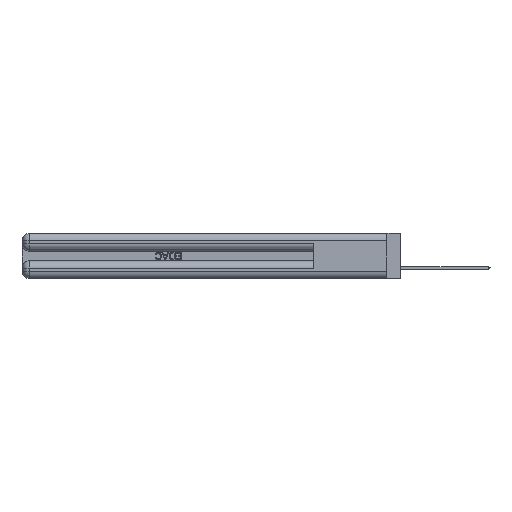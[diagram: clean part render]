
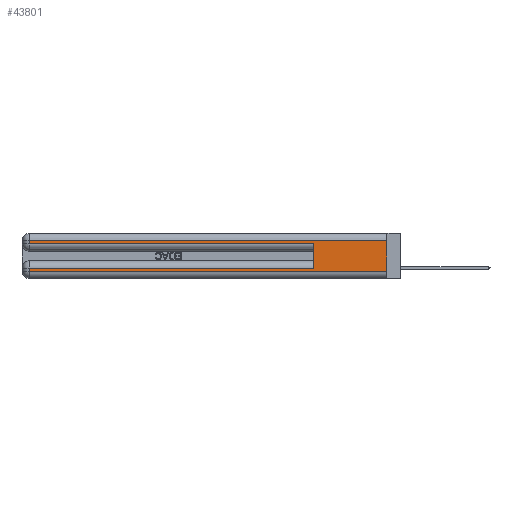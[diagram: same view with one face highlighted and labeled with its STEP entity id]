
A CAD part, left-side view. The second image highlights one B-rep face of the part: STEP entity #43801.
In plain terms, the highlighted planar face has unit normal (-1, 0, 0).
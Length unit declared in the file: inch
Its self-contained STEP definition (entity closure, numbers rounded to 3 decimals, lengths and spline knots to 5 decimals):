
#1832 = DIRECTION ( 'NONE',  ( 0., -1., 0. ) ) ;
#1915 = DIRECTION ( 'NONE',  ( 0., 0., -1. ) ) ;
#3295 = VECTOR ( 'NONE', #17821, 39.37008 ) ;
#3447 = CARTESIAN_POINT ( 'NONE',  ( 0., 0., 0.06 ) ) ;
#3782 = CARTESIAN_POINT ( 'NONE',  ( 0., 0., 0.31 ) ) ;
#4928 = CARTESIAN_POINT ( 'NONE',  ( 0., 2.94, 0.06 ) ) ;
#5348 = VECTOR ( 'NONE', #37592, 39.37008 ) ;
#5986 = CARTESIAN_POINT ( 'NONE',  ( 0., 2.94, 0.37 ) ) ;
#8649 = VECTOR ( 'NONE', #1832, 39.37008 ) ;
#9195 = EDGE_CURVE ( 'NONE', #25537, #36554, #36026, .T. ) ;
#9207 = VECTOR ( 'NONE', #1915, 39.37008 ) ;
#10001 = VERTEX_POINT ( 'NONE', #36965 ) ;
#10470 = VECTOR ( 'NONE', #26512, 39.37008 ) ;
#12424 = VERTEX_POINT ( 'NONE', #3447 ) ;
#13361 = ORIENTED_EDGE ( 'NONE', *, *, #32680, .T. ) ;
#13524 = VERTEX_POINT ( 'NONE', #44220 ) ;
#13766 = CARTESIAN_POINT ( 'NONE',  ( 0., 0.6, 0.145 ) ) ;
#14159 = VERTEX_POINT ( 'NONE', #3782 ) ;
#14842 = EDGE_CURVE ( 'NONE', #36554, #12424, #25068, .T. ) ;
#15254 = FACE_OUTER_BOUND ( 'NONE', #41324, .T. ) ;
#17821 = DIRECTION ( 'NONE',  ( 0., 1., 0. ) ) ;
#19433 = PLANE ( 'NONE',  #24826 ) ;
#21075 = ORIENTED_EDGE ( 'NONE', *, *, #38739, .F. ) ;
#21183 = CARTESIAN_POINT ( 'NONE',  ( 0., 2.94, 0.085 ) ) ;
#21620 = VECTOR ( 'NONE', #30136, 39.37008 ) ;
#21984 = VECTOR ( 'NONE', #36771, 39.37008 ) ;
#22251 = CARTESIAN_POINT ( 'NONE',  ( 0., 0., 0.085 ) ) ;
#22483 = EDGE_CURVE ( 'NONE', #13524, #10001, #26290, .T. ) ;
#22815 = EDGE_CURVE ( 'NONE', #14159, #32329, #37208, .T. ) ;
#23191 = DIRECTION ( 'NONE',  ( 1., 0., 0. ) ) ;
#23272 = ORIENTED_EDGE ( 'NONE', *, *, #9195, .T. ) ;
#23724 = EDGE_CURVE ( 'NONE', #39798, #10001, #25073, .T. ) ;
#24073 = CARTESIAN_POINT ( 'NONE',  ( 0., 0.6, 0.085 ) ) ;
#24826 = AXIS2_PLACEMENT_3D ( 'NONE', #26859, #23191, #40356 ) ;
#25068 = LINE ( 'NONE', #29359, #8649 ) ;
#25073 = LINE ( 'NONE', #13766, #5348 ) ;
#25537 = VERTEX_POINT ( 'NONE', #21183 ) ;
#26290 = LINE ( 'NONE', #32790, #10470 ) ;
#26512 = DIRECTION ( 'NONE',  ( 0., -1., 0. ) ) ;
#26859 = CARTESIAN_POINT ( 'NONE',  ( 0., 0., 0.37 ) ) ;
#27031 = EDGE_CURVE ( 'NONE', #32329, #13524, #30909, .T. ) ;
#27580 = ORIENTED_EDGE ( 'NONE', *, *, #22815, .T. ) ;
#27696 = DIRECTION ( 'NONE',  ( 0., 0., -1. ) ) ;
#28283 = ORIENTED_EDGE ( 'NONE', *, *, #23724, .F. ) ;
#29359 = CARTESIAN_POINT ( 'NONE',  ( 0., 0., 0.06 ) ) ;
#30136 = DIRECTION ( 'NONE',  ( 0., 0., -1. ) ) ;
#30909 = LINE ( 'NONE', #5986, #21620 ) ;
#31129 = LINE ( 'NONE', #31311, #34982 ) ;
#31311 = CARTESIAN_POINT ( 'NONE',  ( 0., 0., 0.37 ) ) ;
#31653 = CARTESIAN_POINT ( 'NONE',  ( 0., 0., 0.31 ) ) ;
#32329 = VERTEX_POINT ( 'NONE', #43645 ) ;
#32680 = EDGE_CURVE ( 'NONE', #39798, #25537, #35688, .T. ) ;
#32790 = CARTESIAN_POINT ( 'NONE',  ( 0., 0., 0.285 ) ) ;
#34100 = ORIENTED_EDGE ( 'NONE', *, *, #27031, .T. ) ;
#34982 = VECTOR ( 'NONE', #27696, 39.37008 ) ;
#35688 = LINE ( 'NONE', #22251, #21984 ) ;
#36026 = LINE ( 'NONE', #38980, #9207 ) ;
#36554 = VERTEX_POINT ( 'NONE', #4928 ) ;
#36771 = DIRECTION ( 'NONE',  ( 0., 1., 0. ) ) ;
#36965 = CARTESIAN_POINT ( 'NONE',  ( 0., 0.6, 0.285 ) ) ;
#37208 = LINE ( 'NONE', #31653, #3295 ) ;
#37592 = DIRECTION ( 'NONE',  ( 0., 0., 1. ) ) ;
#37907 = ORIENTED_EDGE ( 'NONE', *, *, #22483, .T. ) ;
#38739 = EDGE_CURVE ( 'NONE', #14159, #12424, #31129, .T. ) ;
#38980 = CARTESIAN_POINT ( 'NONE',  ( 0., 2.94, 0.37 ) ) ;
#39798 = VERTEX_POINT ( 'NONE', #24073 ) ;
#40356 = DIRECTION ( 'NONE',  ( 0., 0., -1. ) ) ;
#41324 = EDGE_LOOP ( 'NONE', ( #21075, #27580, #34100, #37907, #28283, #13361, #23272, #43988 ) ) ;
#43645 = CARTESIAN_POINT ( 'NONE',  ( 0., 2.94, 0.31 ) ) ;
#43801 = ADVANCED_FACE ( 'NONE', ( #15254 ), #19433, .F. ) ;
#43988 = ORIENTED_EDGE ( 'NONE', *, *, #14842, .T. ) ;
#44220 = CARTESIAN_POINT ( 'NONE',  ( 0., 2.94, 0.285 ) ) ;
